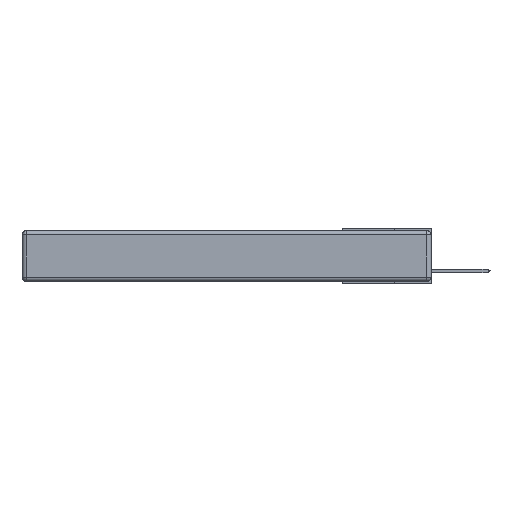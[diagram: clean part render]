
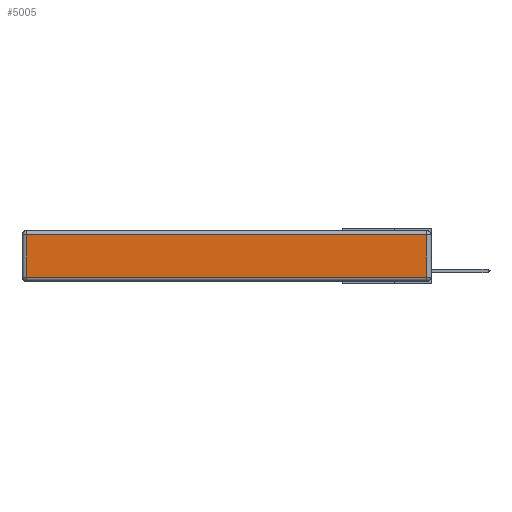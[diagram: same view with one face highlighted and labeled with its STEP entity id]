
A CAD part, left-side view. The second image highlights one B-rep face of the part: STEP entity #5005.
In plain terms, the highlighted planar face has unit normal (-1, 0, 0).
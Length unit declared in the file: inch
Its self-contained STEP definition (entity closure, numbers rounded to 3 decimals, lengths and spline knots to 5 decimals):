
#62 = LINE ( 'NONE', #15470, #4772 ) ;
#728 = VERTEX_POINT ( 'NONE', #6054 ) ;
#829 = EDGE_CURVE ( 'NONE', #9703, #18543, #62, .T. ) ;
#1971 = LINE ( 'NONE', #17060, #14821 ) ;
#2024 = LINE ( 'NONE', #7681, #12234 ) ;
#3502 = AXIS2_PLACEMENT_3D ( 'NONE', #17837, #6001, #19301 ) ;
#3690 = VECTOR ( 'NONE', #18224, 39.37008 ) ;
#4044 = ORIENTED_EDGE ( 'NONE', *, *, #829, .T. ) ;
#4325 = EDGE_CURVE ( 'NONE', #5624, #9703, #2024, .T. ) ;
#4772 = VECTOR ( 'NONE', #10924, 39.37008 ) ;
#4825 = FACE_OUTER_BOUND ( 'NONE', #9817, .T. ) ;
#5005 = ADVANCED_FACE ( 'NONE', ( #4825 ), #7361, .T. ) ;
#5070 = CARTESIAN_POINT ( 'NONE',  ( 0., 2.72, -0.343 ) ) ;
#5232 = DIRECTION ( 'NONE',  ( 0., -1., 0. ) ) ;
#5590 = ORIENTED_EDGE ( 'NONE', *, *, #4325, .T. ) ;
#5624 = VERTEX_POINT ( 'NONE', #8304 ) ;
#6001 = DIRECTION ( 'NONE',  ( -1., 0., 0. ) ) ;
#6054 = CARTESIAN_POINT ( 'NONE',  ( 0., 2.72, -0.313 ) ) ;
#6902 = ORIENTED_EDGE ( 'NONE', *, *, #7409, .T. ) ;
#7338 = ORIENTED_EDGE ( 'NONE', *, *, #12566, .T. ) ;
#7361 = PLANE ( 'NONE',  #3502 ) ;
#7409 = EDGE_CURVE ( 'NONE', #18543, #728, #19930, .T. ) ;
#7681 = CARTESIAN_POINT ( 'NONE',  ( 0., 0.03, -0.343 ) ) ;
#8304 = CARTESIAN_POINT ( 'NONE',  ( 0., 0.03, -0.313 ) ) ;
#9703 = VERTEX_POINT ( 'NONE', #12906 ) ;
#9817 = EDGE_LOOP ( 'NONE', ( #7338, #5590, #4044, #6902 ) ) ;
#10924 = DIRECTION ( 'NONE',  ( 0., 1., 0. ) ) ;
#12234 = VECTOR ( 'NONE', #15101, 39.37008 ) ;
#12566 = EDGE_CURVE ( 'NONE', #728, #5624, #1971, .T. ) ;
#12906 = CARTESIAN_POINT ( 'NONE',  ( 0., 0.03, -0.03 ) ) ;
#14821 = VECTOR ( 'NONE', #5232, 39.37008 ) ;
#15101 = DIRECTION ( 'NONE',  ( 0., 0., 1. ) ) ;
#15292 = CARTESIAN_POINT ( 'NONE',  ( 0., 2.72, -0.03 ) ) ;
#15470 = CARTESIAN_POINT ( 'NONE',  ( 0., 2.75, -0.03 ) ) ;
#17060 = CARTESIAN_POINT ( 'NONE',  ( 0., 0., -0.313 ) ) ;
#17837 = CARTESIAN_POINT ( 'NONE',  ( 0., 0., -0.343 ) ) ;
#18224 = DIRECTION ( 'NONE',  ( 0., 0., -1. ) ) ;
#18543 = VERTEX_POINT ( 'NONE', #15292 ) ;
#19301 = DIRECTION ( 'NONE',  ( 0., 0., 1. ) ) ;
#19930 = LINE ( 'NONE', #5070, #3690 ) ;
